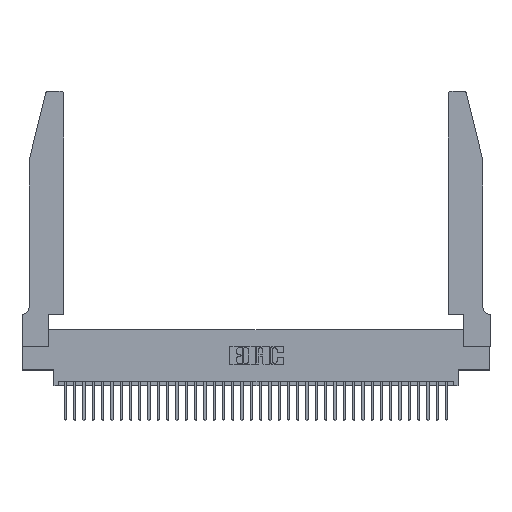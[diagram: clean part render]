
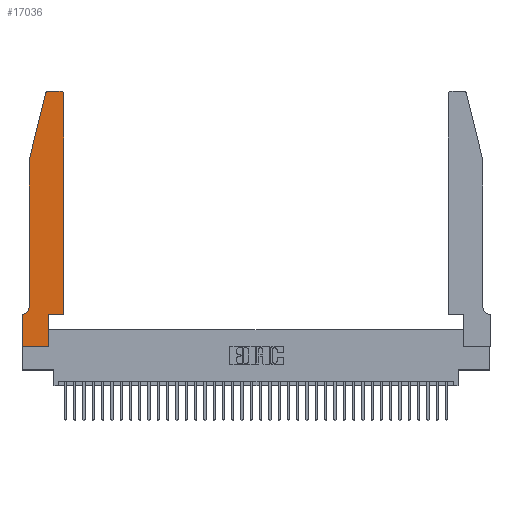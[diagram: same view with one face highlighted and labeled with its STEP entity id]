
A CAD part, top view. The second image highlights one B-rep face of the part: STEP entity #17036.
In plain terms, the highlighted planar face has unit normal (0, 0, 1).
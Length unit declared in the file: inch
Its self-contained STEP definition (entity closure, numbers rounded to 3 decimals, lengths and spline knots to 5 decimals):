
#44 = CARTESIAN_POINT ( 'NONE',  ( 0.2865, 0., 0.37 ) ) ;
#918 = DIRECTION ( 'NONE',  ( 0., 0., 1. ) ) ;
#969 = AXIS2_PLACEMENT_3D ( 'NONE', #18652, #918, #21609 ) ;
#1603 = ORIENTED_EDGE ( 'NONE', *, *, #35352, .T. ) ;
#2342 = VECTOR ( 'NONE', #13930, 39.37008 ) ;
#2492 = DIRECTION ( 'NONE',  ( 0., -1., 0. ) ) ;
#3027 = VECTOR ( 'NONE', #7429, 39.37008 ) ;
#3843 = CARTESIAN_POINT ( 'NONE',  ( 0.4505, 0.35, 0.37 ) ) ;
#4255 = EDGE_CURVE ( 'NONE', #23850, #33647, #10914, .T. ) ;
#4346 = LINE ( 'NONE', #5395, #5286 ) ;
#4623 = VECTOR ( 'NONE', #28255, 39.37008 ) ;
#4671 = AXIS2_PLACEMENT_3D ( 'NONE', #5432, #25983, #8393 ) ;
#4793 = CARTESIAN_POINT ( 'NONE',  ( 0.2865, 0.35, 0.37 ) ) ;
#4856 = VERTEX_POINT ( 'NONE', #22049 ) ;
#5286 = VECTOR ( 'NONE', #8358, 39.37008 ) ;
#5340 = EDGE_CURVE ( 'NONE', #33991, #16947, #15874, .T. ) ;
#5395 = CARTESIAN_POINT ( 'NONE',  ( 0.2605, 2.75, 0.37 ) ) ;
#5432 = CARTESIAN_POINT ( 'NONE',  ( 0.4205, 2.72, 0.37 ) ) ;
#6356 = CARTESIAN_POINT ( 'NONE',  ( 0.0755, 2., 0.37 ) ) ;
#6533 = ORIENTED_EDGE ( 'NONE', *, *, #36118, .T. ) ;
#6853 = DIRECTION ( 'NONE',  ( 0., 0., -1. ) ) ;
#6864 = CARTESIAN_POINT ( 'NONE',  ( 0.0755, 0.35, 0.37 ) ) ;
#7296 = CARTESIAN_POINT ( 'NONE',  ( 0., 0., 0.37 ) ) ;
#7429 = DIRECTION ( 'NONE',  ( 1., 0., 0. ) ) ;
#7475 = CARTESIAN_POINT ( 'NONE',  ( 0.284, 2.75, 0.37 ) ) ;
#7517 = CARTESIAN_POINT ( 'NONE',  ( 0., 0., 0.37 ) ) ;
#8358 = DIRECTION ( 'NONE',  ( -1., 0., 0. ) ) ;
#8393 = DIRECTION ( 'NONE',  ( 1., 0., 0. ) ) ;
#8523 = LINE ( 'NONE', #13548, #30017 ) ;
#8550 = VERTEX_POINT ( 'NONE', #25584 ) ;
#9015 = EDGE_CURVE ( 'NONE', #10529, #23850, #8523, .T. ) ;
#10257 = LINE ( 'NONE', #31379, #2342 ) ;
#10529 = VERTEX_POINT ( 'NONE', #31406 ) ;
#10914 = LINE ( 'NONE', #7296, #3027 ) ;
#11096 = CARTESIAN_POINT ( 'NONE',  ( 0.4505, 0.35, 0.37 ) ) ;
#11098 = VECTOR ( 'NONE', #30265, 39.37008 ) ;
#11215 = AXIS2_PLACEMENT_3D ( 'NONE', #24436, #6853, #27359 ) ;
#12202 = ORIENTED_EDGE ( 'NONE', *, *, #34170, .T. ) ;
#12406 = VECTOR ( 'NONE', #27351, 39.37008 ) ;
#12422 = AXIS2_PLACEMENT_3D ( 'NONE', #13156, #16102, #36395 ) ;
#12965 = LINE ( 'NONE', #6864, #11098 ) ;
#13156 = CARTESIAN_POINT ( 'NONE',  ( 0., 0.35, 0.37 ) ) ;
#13247 = EDGE_CURVE ( 'NONE', #36430, #8550, #35157, .T. ) ;
#13468 = EDGE_CURVE ( 'NONE', #21818, #30748, #28859, .T. ) ;
#13548 = CARTESIAN_POINT ( 'NONE',  ( 0., 0., 0.37 ) ) ;
#13930 = DIRECTION ( 'NONE',  ( -0.239, -0.971, 0. ) ) ;
#14826 = LINE ( 'NONE', #37470, #30333 ) ;
#15874 = CIRCLE ( 'NONE', #969, 0.03 ) ;
#16102 = DIRECTION ( 'NONE',  ( 0., 0., 1. ) ) ;
#16499 = DIRECTION ( 'NONE',  ( 0., -1., 0. ) ) ;
#16947 = VERTEX_POINT ( 'NONE', #18545 ) ;
#17036 = ADVANCED_FACE ( 'NONE', ( #24576 ), #30617, .T. ) ;
#17541 = ORIENTED_EDGE ( 'NONE', *, *, #5340, .T. ) ;
#18545 = CARTESIAN_POINT ( 'NONE',  ( 0.25487, 2.72718, 0.37 ) ) ;
#18652 = CARTESIAN_POINT ( 'NONE',  ( 0.284, 2.72, 0.37 ) ) ;
#19323 = EDGE_CURVE ( 'NONE', #20274, #27901, #14826, .T. ) ;
#19387 = ORIENTED_EDGE ( 'NONE', *, *, #9015, .T. ) ;
#20005 = EDGE_LOOP ( 'NONE', ( #12202, #17541, #1603, #28771, #26112, #6533, #19387, #20295, #20416, #20590, #20787, #32429 ) ) ;
#20274 = VERTEX_POINT ( 'NONE', #6356 ) ;
#20295 = ORIENTED_EDGE ( 'NONE', *, *, #4255, .T. ) ;
#20416 = ORIENTED_EDGE ( 'NONE', *, *, #36340, .T. ) ;
#20590 = ORIENTED_EDGE ( 'NONE', *, *, #13468, .T. ) ;
#20621 = EDGE_CURVE ( 'NONE', #30748, #36430, #33867, .T. ) ;
#20787 = ORIENTED_EDGE ( 'NONE', *, *, #20621, .T. ) ;
#21112 = EDGE_CURVE ( 'NONE', #27901, #4856, #31990, .T. ) ;
#21609 = DIRECTION ( 'NONE',  ( 1., 0., 0. ) ) ;
#21818 = VERTEX_POINT ( 'NONE', #24528 ) ;
#22049 = CARTESIAN_POINT ( 'NONE',  ( 0.0055, 0.35, 0.37 ) ) ;
#23364 = CARTESIAN_POINT ( 'NONE',  ( 0.0755, 0.42, 0.37 ) ) ;
#23850 = VERTEX_POINT ( 'NONE', #7517 ) ;
#24436 = CARTESIAN_POINT ( 'NONE',  ( 0.0055, 0.42, 0.37 ) ) ;
#24528 = CARTESIAN_POINT ( 'NONE',  ( 0.2865, 0.35, 0.37 ) ) ;
#24576 = FACE_OUTER_BOUND ( 'NONE', #20005, .T. ) ;
#25584 = CARTESIAN_POINT ( 'NONE',  ( 0.4205, 2.75, 0.37 ) ) ;
#25717 = DIRECTION ( 'NONE',  ( 0., 1., 0. ) ) ;
#25983 = DIRECTION ( 'NONE',  ( 0., 0., 1. ) ) ;
#26112 = ORIENTED_EDGE ( 'NONE', *, *, #21112, .T. ) ;
#27111 = LINE ( 'NONE', #4793, #4623 ) ;
#27351 = DIRECTION ( 'NONE',  ( 1., 0., 0. ) ) ;
#27359 = DIRECTION ( 'NONE',  ( -1., 0., 0. ) ) ;
#27901 = VERTEX_POINT ( 'NONE', #23364 ) ;
#28255 = DIRECTION ( 'NONE',  ( 0., 1., 0. ) ) ;
#28345 = CARTESIAN_POINT ( 'NONE',  ( 0.4505, 0.35, 0.37 ) ) ;
#28771 = ORIENTED_EDGE ( 'NONE', *, *, #19323, .T. ) ;
#28859 = LINE ( 'NONE', #3843, #12406 ) ;
#30017 = VECTOR ( 'NONE', #16499, 39.37008 ) ;
#30265 = DIRECTION ( 'NONE',  ( -1., 0., 0. ) ) ;
#30333 = VECTOR ( 'NONE', #2492, 39.37008 ) ;
#30617 = PLANE ( 'NONE',  #12422 ) ;
#30748 = VERTEX_POINT ( 'NONE', #28345 ) ;
#31379 = CARTESIAN_POINT ( 'NONE',  ( 0.0755, 2., 0.37 ) ) ;
#31406 = CARTESIAN_POINT ( 'NONE',  ( 0., 0.35, 0.37 ) ) ;
#31990 = CIRCLE ( 'NONE', #11215, 0.07 ) ;
#32429 = ORIENTED_EDGE ( 'NONE', *, *, #13247, .T. ) ;
#32940 = VECTOR ( 'NONE', #25717, 39.37008 ) ;
#33647 = VERTEX_POINT ( 'NONE', #44 ) ;
#33867 = LINE ( 'NONE', #11096, #32940 ) ;
#33991 = VERTEX_POINT ( 'NONE', #7475 ) ;
#34170 = EDGE_CURVE ( 'NONE', #8550, #33991, #4346, .T. ) ;
#35157 = CIRCLE ( 'NONE', #4671, 0.03 ) ;
#35352 = EDGE_CURVE ( 'NONE', #16947, #20274, #10257, .T. ) ;
#36118 = EDGE_CURVE ( 'NONE', #4856, #10529, #12965, .T. ) ;
#36340 = EDGE_CURVE ( 'NONE', #33647, #21818, #27111, .T. ) ;
#36395 = DIRECTION ( 'NONE',  ( 1., 0., 0. ) ) ;
#36430 = VERTEX_POINT ( 'NONE', #37145 ) ;
#37145 = CARTESIAN_POINT ( 'NONE',  ( 0.4505, 2.72, 0.37 ) ) ;
#37470 = CARTESIAN_POINT ( 'NONE',  ( 0.0755, 2., 0.37 ) ) ;
